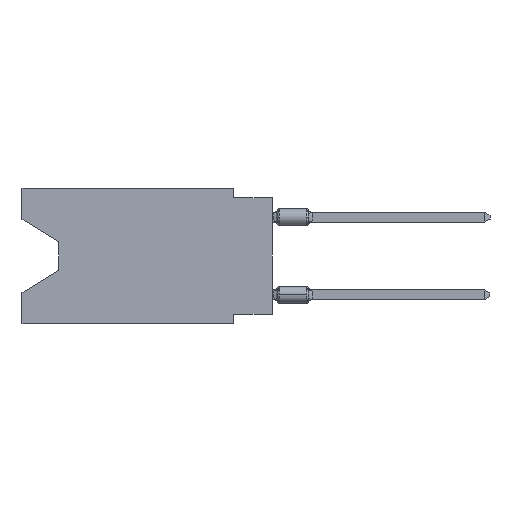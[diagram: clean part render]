
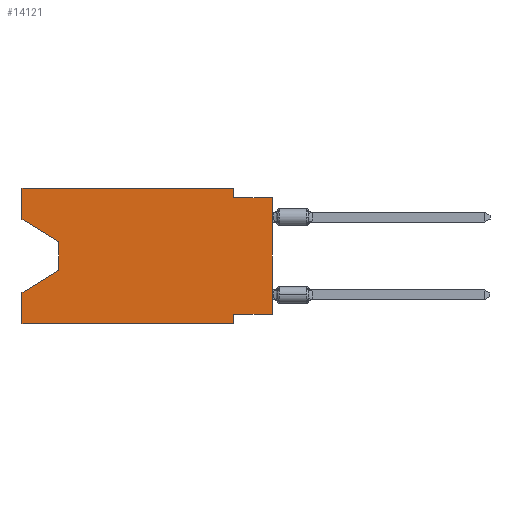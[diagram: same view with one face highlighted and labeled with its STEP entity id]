
A CAD part, left-side view. The second image highlights one B-rep face of the part: STEP entity #14121.
In plain terms, the highlighted planar face has unit normal (-1, 0, 0).
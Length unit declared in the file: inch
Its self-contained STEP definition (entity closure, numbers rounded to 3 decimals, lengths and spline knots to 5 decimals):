
#28 = CARTESIAN_POINT ( 'NONE',  ( 0., 0.55, -0.212 ) ) ;
#36 = ORIENTED_EDGE ( 'NONE', *, *, #4892, .T. ) ;
#68 = CARTESIAN_POINT ( 'NONE',  ( 0., 0., -0.025 ) ) ;
#84 = VERTEX_POINT ( 'NONE', #10423 ) ;
#393 = EDGE_CURVE ( 'NONE', #9301, #10867, #6338, .T. ) ;
#744 = AXIS2_PLACEMENT_3D ( 'NONE', #12506, #3838, #9025 ) ;
#955 = VERTEX_POINT ( 'NONE', #10982 ) ;
#1124 = CARTESIAN_POINT ( 'NONE',  ( 0., 0.645, -0.35 ) ) ;
#1247 = CARTESIAN_POINT ( 'NONE',  ( 0., 0.645, 0. ) ) ;
#1275 = EDGE_CURVE ( 'NONE', #9072, #7999, #11653, .T. ) ;
#1817 = EDGE_CURVE ( 'NONE', #8549, #955, #16086, .T. ) ;
#2100 = ORIENTED_EDGE ( 'NONE', *, *, #14660, .F. ) ;
#2159 = VECTOR ( 'NONE', #5625, 39.37008 ) ;
#2230 = ORIENTED_EDGE ( 'NONE', *, *, #11958, .F. ) ;
#2240 = LINE ( 'NONE', #1124, #3735 ) ;
#2253 = VECTOR ( 'NONE', #12701, 39.37008 ) ;
#2372 = DIRECTION ( 'NONE',  ( 0., 0., 1. ) ) ;
#2405 = DIRECTION ( 'NONE',  ( 0., 1., 0. ) ) ;
#2748 = CARTESIAN_POINT ( 'NONE',  ( 0., 0.55, -0.138 ) ) ;
#2804 = CARTESIAN_POINT ( 'NONE',  ( 0., 0.645, -0.08025 ) ) ;
#3234 = DIRECTION ( 'NONE',  ( 0., 0., 1. ) ) ;
#3408 = LINE ( 'NONE', #13783, #5814 ) ;
#3735 = VECTOR ( 'NONE', #15245, 39.37008 ) ;
#3826 = VECTOR ( 'NONE', #13373, 39.37008 ) ;
#3838 = DIRECTION ( 'NONE',  ( 1., 0., 0. ) ) ;
#3920 = LINE ( 'NONE', #14637, #2159 ) ;
#4591 = LINE ( 'NONE', #14886, #15079 ) ;
#4892 = EDGE_CURVE ( 'NONE', #6217, #10867, #2240, .T. ) ;
#5250 = LINE ( 'NONE', #1247, #6818 ) ;
#5625 = DIRECTION ( 'NONE',  ( 0., 0., 1. ) ) ;
#5651 = CARTESIAN_POINT ( 'NONE',  ( 0., 0.1, 0. ) ) ;
#5814 = VECTOR ( 'NONE', #15146, 39.37008 ) ;
#5879 = ORIENTED_EDGE ( 'NONE', *, *, #15513, .F. ) ;
#6217 = VERTEX_POINT ( 'NONE', #15659 ) ;
#6221 = EDGE_CURVE ( 'NONE', #84, #12734, #3920, .T. ) ;
#6338 = LINE ( 'NONE', #14066, #2253 ) ;
#6438 = DIRECTION ( 'NONE',  ( 0., -1., 0. ) ) ;
#6818 = VECTOR ( 'NONE', #2372, 39.37008 ) ;
#7216 = VECTOR ( 'NONE', #7932, 39.37008 ) ;
#7544 = ORIENTED_EDGE ( 'NONE', *, *, #11258, .F. ) ;
#7667 = LINE ( 'NONE', #8859, #7689 ) ;
#7689 = VECTOR ( 'NONE', #2405, 39.37008 ) ;
#7873 = VERTEX_POINT ( 'NONE', #13678 ) ;
#7932 = DIRECTION ( 'NONE',  ( 0., 0., -1. ) ) ;
#7999 = VERTEX_POINT ( 'NONE', #13052 ) ;
#8549 = VERTEX_POINT ( 'NONE', #5651 ) ;
#8585 = ORIENTED_EDGE ( 'NONE', *, *, #6221, .T. ) ;
#8797 = ORIENTED_EDGE ( 'NONE', *, *, #12646, .T. ) ;
#8859 = CARTESIAN_POINT ( 'NONE',  ( 0., 0., -0.325 ) ) ;
#9025 = DIRECTION ( 'NONE',  ( 0., 0., -1. ) ) ;
#9072 = VERTEX_POINT ( 'NONE', #11142 ) ;
#9230 = ORIENTED_EDGE ( 'NONE', *, *, #1817, .F. ) ;
#9301 = VERTEX_POINT ( 'NONE', #11788 ) ;
#9373 = CARTESIAN_POINT ( 'NONE',  ( 0., 0.645, 0. ) ) ;
#9421 = VECTOR ( 'NONE', #6438, 39.37008 ) ;
#9604 = CARTESIAN_POINT ( 'NONE',  ( 0., 0.1, 0. ) ) ;
#9936 = VERTEX_POINT ( 'NONE', #12271 ) ;
#10423 = CARTESIAN_POINT ( 'NONE',  ( 0., 0., -0.325 ) ) ;
#10519 = VERTEX_POINT ( 'NONE', #2804 ) ;
#10867 = VERTEX_POINT ( 'NONE', #11523 ) ;
#10982 = CARTESIAN_POINT ( 'NONE',  ( 0., 0.1, -0.025 ) ) ;
#11142 = CARTESIAN_POINT ( 'NONE',  ( 0., 0.55, -0.212 ) ) ;
#11258 = EDGE_CURVE ( 'NONE', #7873, #8549, #14401, .T. ) ;
#11318 = VECTOR ( 'NONE', #15758, 39.37008 ) ;
#11352 = ORIENTED_EDGE ( 'NONE', *, *, #16099, .F. ) ;
#11506 = ORIENTED_EDGE ( 'NONE', *, *, #16504, .T. ) ;
#11523 = CARTESIAN_POINT ( 'NONE',  ( 0., 0.1, -0.35 ) ) ;
#11653 = LINE ( 'NONE', #28, #11318 ) ;
#11788 = CARTESIAN_POINT ( 'NONE',  ( 0., 0.1, -0.325 ) ) ;
#11958 = EDGE_CURVE ( 'NONE', #6217, #7999, #5250, .T. ) ;
#12271 = CARTESIAN_POINT ( 'NONE',  ( 0., 0.55, -0.138 ) ) ;
#12396 = EDGE_LOOP ( 'NONE', ( #11506, #8797, #13756, #2230, #36, #16497, #11352, #8585, #2100, #9230, #7544, #5879 ) ) ;
#12506 = CARTESIAN_POINT ( 'NONE',  ( 0., 0.645, 0. ) ) ;
#12646 = EDGE_CURVE ( 'NONE', #9936, #9072, #15761, .T. ) ;
#12701 = DIRECTION ( 'NONE',  ( 0., 0., -1. ) ) ;
#12734 = VERTEX_POINT ( 'NONE', #13443 ) ;
#12889 = LINE ( 'NONE', #68, #9421 ) ;
#13045 = VECTOR ( 'NONE', #15302, 39.37008 ) ;
#13052 = CARTESIAN_POINT ( 'NONE',  ( 0., 0.645, -0.26975 ) ) ;
#13373 = DIRECTION ( 'NONE',  ( 0., -1., 0. ) ) ;
#13443 = CARTESIAN_POINT ( 'NONE',  ( 0., 0., -0.025 ) ) ;
#13678 = CARTESIAN_POINT ( 'NONE',  ( 0., 0.645, 0. ) ) ;
#13756 = ORIENTED_EDGE ( 'NONE', *, *, #1275, .T. ) ;
#13783 = CARTESIAN_POINT ( 'NONE',  ( 0., 0.645, -0.08025 ) ) ;
#13880 = PLANE ( 'NONE',  #744 ) ;
#14066 = CARTESIAN_POINT ( 'NONE',  ( 0., 0.1, -0.35 ) ) ;
#14121 = ADVANCED_FACE ( 'NONE', ( #15492 ), #13880, .F. ) ;
#14401 = LINE ( 'NONE', #9373, #3826 ) ;
#14637 = CARTESIAN_POINT ( 'NONE',  ( 0., 0., 0. ) ) ;
#14660 = EDGE_CURVE ( 'NONE', #955, #12734, #12889, .T. ) ;
#14886 = CARTESIAN_POINT ( 'NONE',  ( 0., 0.645, 0. ) ) ;
#15079 = VECTOR ( 'NONE', #3234, 39.37008 ) ;
#15146 = DIRECTION ( 'NONE',  ( 0., -0.855, -0.519 ) ) ;
#15245 = DIRECTION ( 'NONE',  ( 0., -1., 0. ) ) ;
#15302 = DIRECTION ( 'NONE',  ( 0., 0., -1. ) ) ;
#15492 = FACE_OUTER_BOUND ( 'NONE', #12396, .T. ) ;
#15513 = EDGE_CURVE ( 'NONE', #10519, #7873, #4591, .T. ) ;
#15659 = CARTESIAN_POINT ( 'NONE',  ( 0., 0.645, -0.35 ) ) ;
#15758 = DIRECTION ( 'NONE',  ( 0., 0.855, -0.519 ) ) ;
#15761 = LINE ( 'NONE', #2748, #7216 ) ;
#16086 = LINE ( 'NONE', #9604, #13045 ) ;
#16099 = EDGE_CURVE ( 'NONE', #84, #9301, #7667, .T. ) ;
#16497 = ORIENTED_EDGE ( 'NONE', *, *, #393, .F. ) ;
#16504 = EDGE_CURVE ( 'NONE', #10519, #9936, #3408, .T. ) ;
